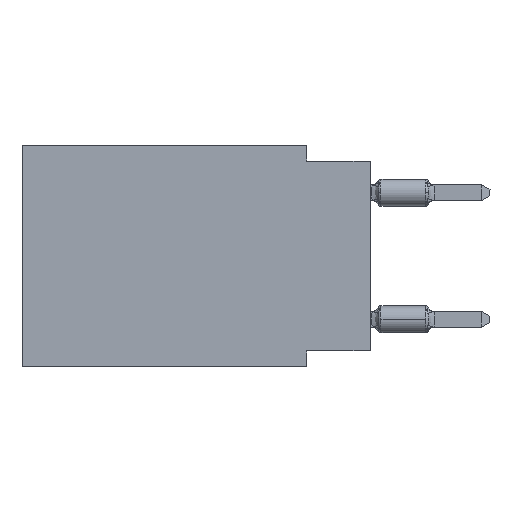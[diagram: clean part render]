
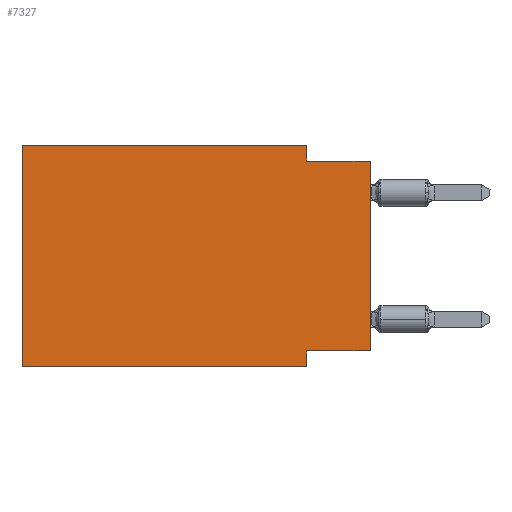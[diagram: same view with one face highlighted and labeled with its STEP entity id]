
A CAD part, left-side view. The second image highlights one B-rep face of the part: STEP entity #7327.
In plain terms, the highlighted planar face has unit normal (-1, 0, 0).
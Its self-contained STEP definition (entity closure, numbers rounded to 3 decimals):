
#222 = ORIENTED_EDGE ( 'NONE', *, *, #371, .F. ) ;
#371 = EDGE_CURVE ( 'NONE', #1273, #6929, #3013, .T. ) ;
#677 = LINE ( 'NONE', #14635, #6161 ) ;
#752 = EDGE_CURVE ( 'NONE', #9734, #5865, #8881, .T. ) ;
#804 = CARTESIAN_POINT ( 'NONE',  ( 0., 13.97, 0. ) ) ;
#891 = ORIENTED_EDGE ( 'NONE', *, *, #3234, .T. ) ;
#1273 = VERTEX_POINT ( 'NONE', #3635 ) ;
#1492 = VECTOR ( 'NONE', #8978, 1000. ) ;
#1609 = CARTESIAN_POINT ( 'NONE',  ( 0., 13.97, 0. ) ) ;
#1942 = CARTESIAN_POINT ( 'NONE',  ( 0., 0., -8.255 ) ) ;
#2137 = LINE ( 'NONE', #13785, #6735 ) ;
#2219 = VECTOR ( 'NONE', #2283, 1000. ) ;
#2283 = DIRECTION ( 'NONE',  ( 0., -1., 0. ) ) ;
#2396 = EDGE_CURVE ( 'NONE', #8668, #9734, #677, .T. ) ;
#2646 = ORIENTED_EDGE ( 'NONE', *, *, #8045, .F. ) ;
#2949 = VERTEX_POINT ( 'NONE', #3551 ) ;
#3013 = LINE ( 'NONE', #1942, #1492 ) ;
#3234 = EDGE_CURVE ( 'NONE', #1273, #10823, #7744, .T. ) ;
#3551 = CARTESIAN_POINT ( 'NONE',  ( 0., 13.97, -8.89 ) ) ;
#3606 = EDGE_CURVE ( 'NONE', #6929, #14732, #10781, .T. ) ;
#3635 = CARTESIAN_POINT ( 'NONE',  ( 0., 0., -8.255 ) ) ;
#4026 = DIRECTION ( 'NONE',  ( 1., 0., 0. ) ) ;
#4290 = DIRECTION ( 'NONE',  ( 0., 0., -1. ) ) ;
#4708 = VECTOR ( 'NONE', #13729, 1000. ) ;
#4757 = ORIENTED_EDGE ( 'NONE', *, *, #7164, .F. ) ;
#4818 = DIRECTION ( 'NONE',  ( 0., -1., 0. ) ) ;
#4893 = LINE ( 'NONE', #5976, #13422 ) ;
#4947 = DIRECTION ( 'NONE',  ( 0., 0., -1. ) ) ;
#5340 = ORIENTED_EDGE ( 'NONE', *, *, #3606, .F. ) ;
#5355 = CARTESIAN_POINT ( 'NONE',  ( 0., 2.54, 0. ) ) ;
#5397 = VECTOR ( 'NONE', #4290, 1000. ) ;
#5865 = VERTEX_POINT ( 'NONE', #10956 ) ;
#5976 = CARTESIAN_POINT ( 'NONE',  ( 0., 0., -0.635 ) ) ;
#6161 = VECTOR ( 'NONE', #14563, 1000. ) ;
#6166 = CARTESIAN_POINT ( 'NONE',  ( 0., 2.54, -8.89 ) ) ;
#6735 = VECTOR ( 'NONE', #6789, 1000. ) ;
#6789 = DIRECTION ( 'NONE',  ( 0., 0., 1. ) ) ;
#6929 = VERTEX_POINT ( 'NONE', #9045 ) ;
#7084 = CARTESIAN_POINT ( 'NONE',  ( 0., 13.97, -8.89 ) ) ;
#7164 = EDGE_CURVE ( 'NONE', #2949, #8668, #2137, .T. ) ;
#7327 = ADVANCED_FACE ( 'NONE', ( #11986 ), #12366, .F. ) ;
#7744 = LINE ( 'NONE', #8890, #4708 ) ;
#8045 = EDGE_CURVE ( 'NONE', #5865, #10823, #4893, .T. ) ;
#8166 = LINE ( 'NONE', #7084, #2219 ) ;
#8253 = CARTESIAN_POINT ( 'NONE',  ( 0., 2.54, 0. ) ) ;
#8668 = VERTEX_POINT ( 'NONE', #1609 ) ;
#8881 = LINE ( 'NONE', #5355, #5397 ) ;
#8890 = CARTESIAN_POINT ( 'NONE',  ( 0., 0., 0. ) ) ;
#8978 = DIRECTION ( 'NONE',  ( 0., 1., 0. ) ) ;
#9045 = CARTESIAN_POINT ( 'NONE',  ( 0., 2.54, -8.255 ) ) ;
#9330 = CARTESIAN_POINT ( 'NONE',  ( 0., 0., -0.635 ) ) ;
#9734 = VERTEX_POINT ( 'NONE', #8253 ) ;
#10074 = EDGE_CURVE ( 'NONE', #2949, #14732, #8166, .T. ) ;
#10781 = LINE ( 'NONE', #6166, #12798 ) ;
#10823 = VERTEX_POINT ( 'NONE', #9330 ) ;
#10956 = CARTESIAN_POINT ( 'NONE',  ( 0., 2.54, -0.635 ) ) ;
#11073 = DIRECTION ( 'NONE',  ( 0., 0., -1. ) ) ;
#11887 = AXIS2_PLACEMENT_3D ( 'NONE', #804, #4026, #11073 ) ;
#11986 = FACE_OUTER_BOUND ( 'NONE', #14624, .T. ) ;
#12366 = PLANE ( 'NONE',  #11887 ) ;
#12798 = VECTOR ( 'NONE', #4947, 1000. ) ;
#13422 = VECTOR ( 'NONE', #4818, 1000. ) ;
#13578 = CARTESIAN_POINT ( 'NONE',  ( 0., 2.54, -8.89 ) ) ;
#13602 = ORIENTED_EDGE ( 'NONE', *, *, #752, .F. ) ;
#13729 = DIRECTION ( 'NONE',  ( 0., 0., 1. ) ) ;
#13785 = CARTESIAN_POINT ( 'NONE',  ( 0., 13.97, 0. ) ) ;
#13923 = ORIENTED_EDGE ( 'NONE', *, *, #2396, .F. ) ;
#13961 = ORIENTED_EDGE ( 'NONE', *, *, #10074, .T. ) ;
#14563 = DIRECTION ( 'NONE',  ( 0., -1., 0. ) ) ;
#14624 = EDGE_LOOP ( 'NONE', ( #891, #2646, #13602, #13923, #4757, #13961, #5340, #222 ) ) ;
#14635 = CARTESIAN_POINT ( 'NONE',  ( 0., 13.97, 0. ) ) ;
#14732 = VERTEX_POINT ( 'NONE', #13578 ) ;
